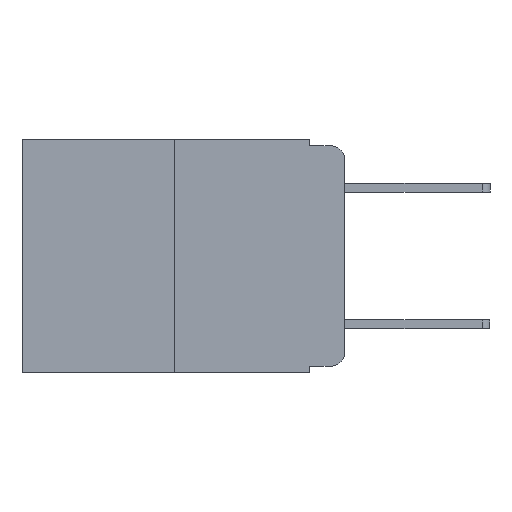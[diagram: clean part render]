
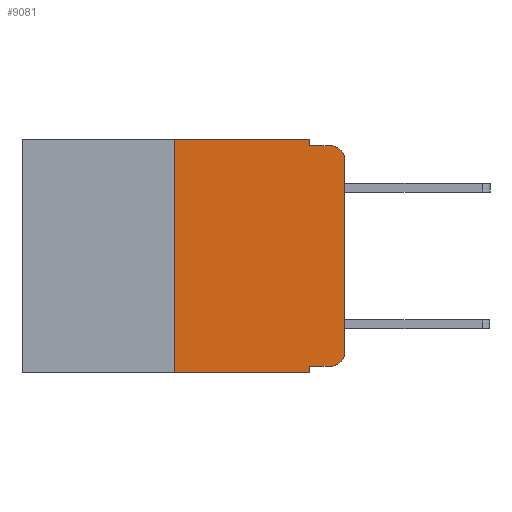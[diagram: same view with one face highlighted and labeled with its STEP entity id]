
A CAD part, left-side view. The second image highlights one B-rep face of the part: STEP entity #9081.
In plain terms, the highlighted planar face has unit normal (-1, 0, 0).
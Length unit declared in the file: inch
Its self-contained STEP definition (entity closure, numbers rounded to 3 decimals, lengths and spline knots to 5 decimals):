
#79 = AXIS2_PLACEMENT_3D ( 'NONE', #2947, #13212, #4432 ) ;
#264 = DIRECTION ( 'NONE',  ( 0., -1., 0. ) ) ;
#284 = VERTEX_POINT ( 'NONE', #8615 ) ;
#352 = CARTESIAN_POINT ( 'NONE',  ( 0., 0.473, 0. ) ) ;
#489 = ORIENTED_EDGE ( 'NONE', *, *, #2388, .T. ) ;
#655 = FACE_OUTER_BOUND ( 'NONE', #6606, .T. ) ;
#857 = DIRECTION ( 'NONE',  ( -1., 0., 0. ) ) ;
#908 = VECTOR ( 'NONE', #17412, 39.37008 ) ;
#1173 = ORIENTED_EDGE ( 'NONE', *, *, #2414, .F. ) ;
#1367 = LINE ( 'NONE', #15952, #908 ) ;
#1665 = LINE ( 'NONE', #10269, #5545 ) ;
#1674 = CARTESIAN_POINT ( 'NONE',  ( 0., 0.25, 0. ) ) ;
#1805 = DIRECTION ( 'NONE',  ( 0., 0., -1. ) ) ;
#2024 = EDGE_CURVE ( 'NONE', #16752, #5579, #1665, .T. ) ;
#2388 = EDGE_CURVE ( 'NONE', #10137, #284, #17939, .T. ) ;
#2414 = EDGE_CURVE ( 'NONE', #9653, #16752, #17476, .T. ) ;
#2638 = AXIS2_PLACEMENT_3D ( 'NONE', #9611, #857, #11094 ) ;
#2756 = VECTOR ( 'NONE', #17728, 39.37008 ) ;
#2828 = VECTOR ( 'NONE', #12377, 39.37008 ) ;
#2947 = CARTESIAN_POINT ( 'NONE',  ( 0., 0.02, -0.313 ) ) ;
#3010 = CARTESIAN_POINT ( 'NONE',  ( 0., 0.25, 0. ) ) ;
#3033 = VECTOR ( 'NONE', #12118, 39.37008 ) ;
#3070 = CARTESIAN_POINT ( 'NONE',  ( 0., 0.051, -0.01 ) ) ;
#3328 = CARTESIAN_POINT ( 'NONE',  ( 0., 0.051, -0.333 ) ) ;
#3630 = AXIS2_PLACEMENT_3D ( 'NONE', #352, #10579, #1805 ) ;
#4432 = DIRECTION ( 'NONE',  ( 0., 0., -1. ) ) ;
#4570 = CARTESIAN_POINT ( 'NONE',  ( 0., 0.02, -0.333 ) ) ;
#4611 = DIRECTION ( 'NONE',  ( 0., 0., -1. ) ) ;
#4613 = DIRECTION ( 'NONE',  ( 0., 0., 1. ) ) ;
#5053 = VERTEX_POINT ( 'NONE', #4570 ) ;
#5068 = VERTEX_POINT ( 'NONE', #13363 ) ;
#5213 = EDGE_CURVE ( 'NONE', #9599, #9653, #8681, .T. ) ;
#5257 = ORIENTED_EDGE ( 'NONE', *, *, #18449, .T. ) ;
#5513 = ORIENTED_EDGE ( 'NONE', *, *, #18531, .T. ) ;
#5545 = VECTOR ( 'NONE', #264, 39.37008 ) ;
#5568 = LINE ( 'NONE', #1674, #12938 ) ;
#5579 = VERTEX_POINT ( 'NONE', #14569 ) ;
#6299 = DIRECTION ( 'NONE',  ( 0., -1., 0. ) ) ;
#6450 = CARTESIAN_POINT ( 'NONE',  ( 0., 0.051, 0. ) ) ;
#6606 = EDGE_LOOP ( 'NONE', ( #489, #18102, #9199, #1173, #9208, #14487, #5513, #7873, #16499, #5257 ) ) ;
#7517 = CARTESIAN_POINT ( 'NONE',  ( 0., 0., -0.313 ) ) ;
#7873 = ORIENTED_EDGE ( 'NONE', *, *, #16057, .F. ) ;
#8615 = CARTESIAN_POINT ( 'NONE',  ( 0., 0., -0.03 ) ) ;
#8655 = CIRCLE ( 'NONE', #2638, 0.02 ) ;
#8681 = LINE ( 'NONE', #13747, #15538 ) ;
#8964 = CARTESIAN_POINT ( 'NONE',  ( 0., 0.473, -0.343 ) ) ;
#9081 = ADVANCED_FACE ( 'NONE', ( #655 ), #16404, .F. ) ;
#9199 = ORIENTED_EDGE ( 'NONE', *, *, #2024, .F. ) ;
#9208 = ORIENTED_EDGE ( 'NONE', *, *, #5213, .F. ) ;
#9599 = VERTEX_POINT ( 'NONE', #3010 ) ;
#9611 = CARTESIAN_POINT ( 'NONE',  ( 0., 0.02, -0.03 ) ) ;
#9653 = VERTEX_POINT ( 'NONE', #11924 ) ;
#10085 = LINE ( 'NONE', #8964, #2756 ) ;
#10137 = VERTEX_POINT ( 'NONE', #7517 ) ;
#10269 = CARTESIAN_POINT ( 'NONE',  ( 0., 0.051, -0.01 ) ) ;
#10386 = EDGE_CURVE ( 'NONE', #284, #5579, #8655, .T. ) ;
#10579 = DIRECTION ( 'NONE',  ( 1., 0., 0. ) ) ;
#11094 = DIRECTION ( 'NONE',  ( 0., 0., -1. ) ) ;
#11924 = CARTESIAN_POINT ( 'NONE',  ( 0., 0.051, 0. ) ) ;
#12118 = DIRECTION ( 'NONE',  ( 0., -1., 0. ) ) ;
#12377 = DIRECTION ( 'NONE',  ( 0., 0., 1. ) ) ;
#12620 = EDGE_CURVE ( 'NONE', #5068, #9599, #5568, .T. ) ;
#12938 = VECTOR ( 'NONE', #4613, 39.37008 ) ;
#13212 = DIRECTION ( 'NONE',  ( -1., 0., 0. ) ) ;
#13363 = CARTESIAN_POINT ( 'NONE',  ( 0., 0.25, -0.343 ) ) ;
#13747 = CARTESIAN_POINT ( 'NONE',  ( 0., 0.473, 0. ) ) ;
#14294 = LINE ( 'NONE', #3328, #3033 ) ;
#14295 = VERTEX_POINT ( 'NONE', #17549 ) ;
#14453 = EDGE_CURVE ( 'NONE', #16340, #5053, #14294, .T. ) ;
#14487 = ORIENTED_EDGE ( 'NONE', *, *, #12620, .F. ) ;
#14569 = CARTESIAN_POINT ( 'NONE',  ( 0., 0.02, -0.01 ) ) ;
#15367 = CIRCLE ( 'NONE', #79, 0.02 ) ;
#15538 = VECTOR ( 'NONE', #6299, 39.37008 ) ;
#15952 = CARTESIAN_POINT ( 'NONE',  ( 0., 0.051, 0. ) ) ;
#16057 = EDGE_CURVE ( 'NONE', #16340, #14295, #1367, .T. ) ;
#16340 = VERTEX_POINT ( 'NONE', #18297 ) ;
#16404 = PLANE ( 'NONE',  #3630 ) ;
#16499 = ORIENTED_EDGE ( 'NONE', *, *, #14453, .T. ) ;
#16752 = VERTEX_POINT ( 'NONE', #3070 ) ;
#17412 = DIRECTION ( 'NONE',  ( 0., 0., -1. ) ) ;
#17476 = LINE ( 'NONE', #6450, #18388 ) ;
#17549 = CARTESIAN_POINT ( 'NONE',  ( 0., 0.051, -0.343 ) ) ;
#17728 = DIRECTION ( 'NONE',  ( 0., -1., 0. ) ) ;
#17939 = LINE ( 'NONE', #18847, #2828 ) ;
#18102 = ORIENTED_EDGE ( 'NONE', *, *, #10386, .T. ) ;
#18297 = CARTESIAN_POINT ( 'NONE',  ( 0., 0.051, -0.333 ) ) ;
#18388 = VECTOR ( 'NONE', #4611, 39.37008 ) ;
#18449 = EDGE_CURVE ( 'NONE', #5053, #10137, #15367, .T. ) ;
#18531 = EDGE_CURVE ( 'NONE', #5068, #14295, #10085, .T. ) ;
#18847 = CARTESIAN_POINT ( 'NONE',  ( 0., 0., 0. ) ) ;
